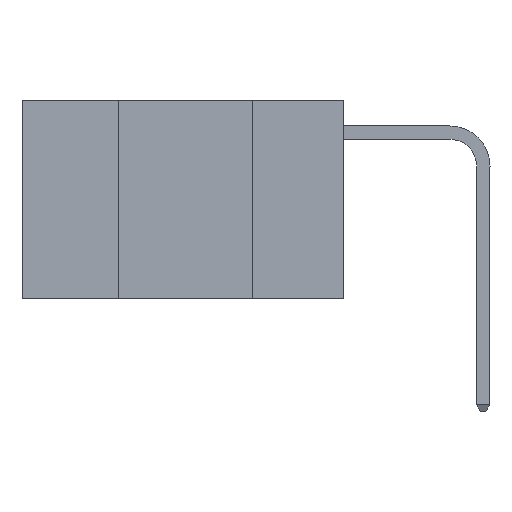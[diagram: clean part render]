
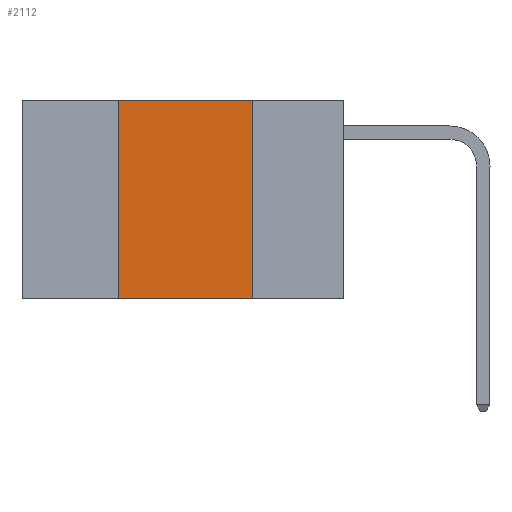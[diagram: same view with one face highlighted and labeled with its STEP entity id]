
A CAD part, left-side view. The second image highlights one B-rep face of the part: STEP entity #2112.
In plain terms, the highlighted planar face has unit normal (-1, 0, 0).
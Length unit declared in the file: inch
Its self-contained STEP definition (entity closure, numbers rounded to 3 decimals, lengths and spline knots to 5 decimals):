
#509 = EDGE_CURVE ( 'NONE', #12711, #12536, #5129, .T. ) ;
#1014 = CARTESIAN_POINT ( 'NONE',  ( 0., 0.42, 0. ) ) ;
#1595 = VECTOR ( 'NONE', #6012, 39.37008 ) ;
#1810 = VECTOR ( 'NONE', #13439, 39.37008 ) ;
#2112 = ADVANCED_FACE ( 'NONE', ( #3708 ), #6300, .F. ) ;
#2212 = VERTEX_POINT ( 'NONE', #15444 ) ;
#2250 = VECTOR ( 'NONE', #14222, 39.37008 ) ;
#3708 = FACE_OUTER_BOUND ( 'NONE', #15504, .T. ) ;
#3818 = CARTESIAN_POINT ( 'NONE',  ( 0., 0.6, 0. ) ) ;
#4923 = LINE ( 'NONE', #1014, #1595 ) ;
#5129 = LINE ( 'NONE', #5667, #1810 ) ;
#5560 = CARTESIAN_POINT ( 'NONE',  ( 0., 0.42, -0.37 ) ) ;
#5667 = CARTESIAN_POINT ( 'NONE',  ( 0., 0.6, -0.37 ) ) ;
#6012 = DIRECTION ( 'NONE',  ( 0., 0., 1. ) ) ;
#6132 = VERTEX_POINT ( 'NONE', #15446 ) ;
#6229 = DIRECTION ( 'NONE',  ( 0., 0., -1. ) ) ;
#6247 = DIRECTION ( 'NONE',  ( 1., 0., 0. ) ) ;
#6300 = PLANE ( 'NONE',  #8798 ) ;
#6304 = CARTESIAN_POINT ( 'NONE',  ( 0., 0.6, 0. ) ) ;
#8088 = ORIENTED_EDGE ( 'NONE', *, *, #509, .T. ) ;
#8678 = LINE ( 'NONE', #13082, #2250 ) ;
#8798 = AXIS2_PLACEMENT_3D ( 'NONE', #6304, #6247, #6229 ) ;
#9338 = ORIENTED_EDGE ( 'NONE', *, *, #13005, .F. ) ;
#9693 = CARTESIAN_POINT ( 'NONE',  ( 0., 0.17, -0.37 ) ) ;
#12311 = LINE ( 'NONE', #3818, #14265 ) ;
#12521 = ORIENTED_EDGE ( 'NONE', *, *, #15279, .F. ) ;
#12536 = VERTEX_POINT ( 'NONE', #9693 ) ;
#12711 = VERTEX_POINT ( 'NONE', #5560 ) ;
#13005 = EDGE_CURVE ( 'NONE', #6132, #2212, #12311, .T. ) ;
#13082 = CARTESIAN_POINT ( 'NONE',  ( 0., 0.17, 0. ) ) ;
#13222 = DIRECTION ( 'NONE',  ( 0., -1., 0. ) ) ;
#13439 = DIRECTION ( 'NONE',  ( 0., -1., 0. ) ) ;
#14222 = DIRECTION ( 'NONE',  ( 0., 0., -1. ) ) ;
#14265 = VECTOR ( 'NONE', #13222, 39.37008 ) ;
#14520 = EDGE_CURVE ( 'NONE', #2212, #12536, #8678, .T. ) ;
#14716 = ORIENTED_EDGE ( 'NONE', *, *, #14520, .F. ) ;
#15279 = EDGE_CURVE ( 'NONE', #12711, #6132, #4923, .T. ) ;
#15444 = CARTESIAN_POINT ( 'NONE',  ( 0., 0.17, 0. ) ) ;
#15446 = CARTESIAN_POINT ( 'NONE',  ( 0., 0.42, 0. ) ) ;
#15504 = EDGE_LOOP ( 'NONE', ( #14716, #9338, #12521, #8088 ) ) ;
